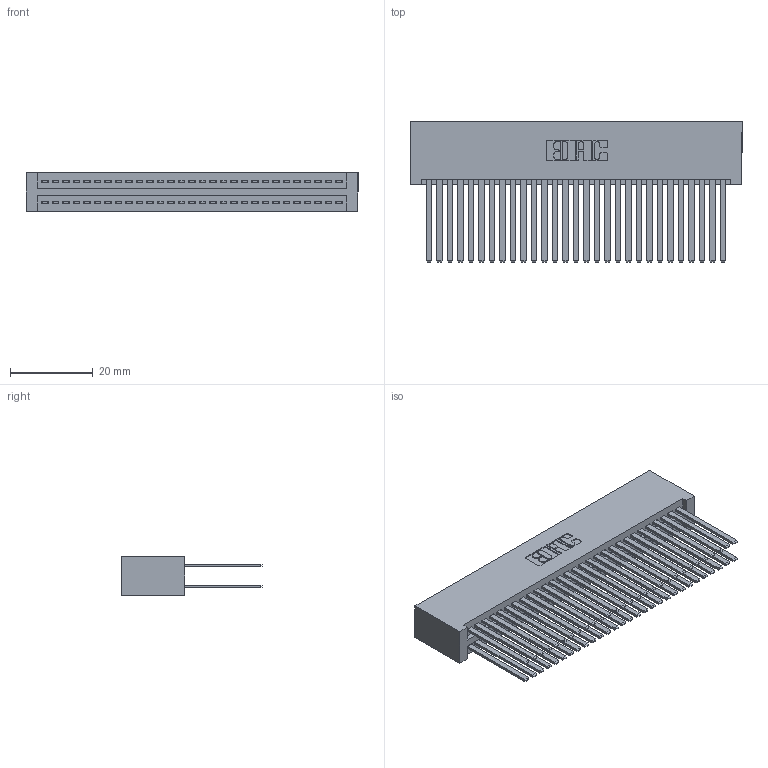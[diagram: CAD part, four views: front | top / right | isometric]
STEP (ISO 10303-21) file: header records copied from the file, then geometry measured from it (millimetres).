
FILE_DESCRIPTION (( 'STEP AP203' ), '1' );
FILE_NAME ('345-058-544-201.STEP', '2019-10-30T05:38:37', ( '' ), ( '' ), 'SwSTEP 2.0', 'SolidWorks 2016', '' );
FILE_SCHEMA (( 'CONFIG_CONTROL_DESIGN' ));
Length unit declared in the file: inch
Products named in the file (3): 345-292-001_345-293-144; 345-058-544-201; 345 Part_No Mounting Lugs
Assembly tree (59 placements, depth 2):
  345-058-544-201
    345 Part_No Mounting Lugs
    345-292-001_345-293-144  x58
Bounding box: 80.26 x 33.96 x 9.4 mm (x, y, z)
Volume: 9105.2 mm3; surface area: 15893.5 mm2
Topology: 59 solids, 59 shells, 2670 faces, 7915 edges, 5198 vertices
Faces by surface type: plane 1758, cylinder 912
Entity records: 24043 total; most frequent: CARTESIAN_POINT 4040, ORIENTED_EDGE 3974, DIRECTION 3571, EDGE_CURVE 1987, LINE 1751, VECTOR 1751, VERTEX_POINT 1322, AXIS2_PLACEMENT_3D 910
